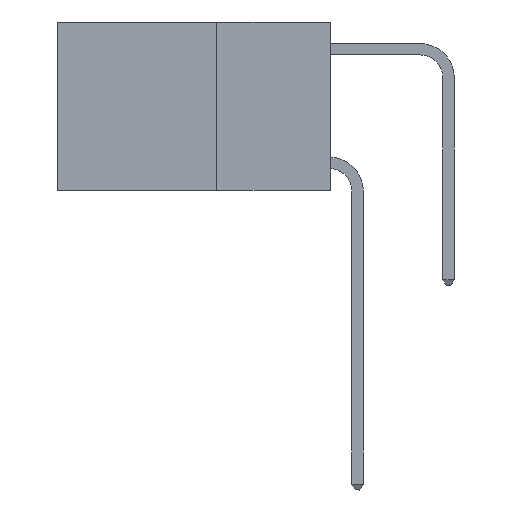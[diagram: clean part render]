
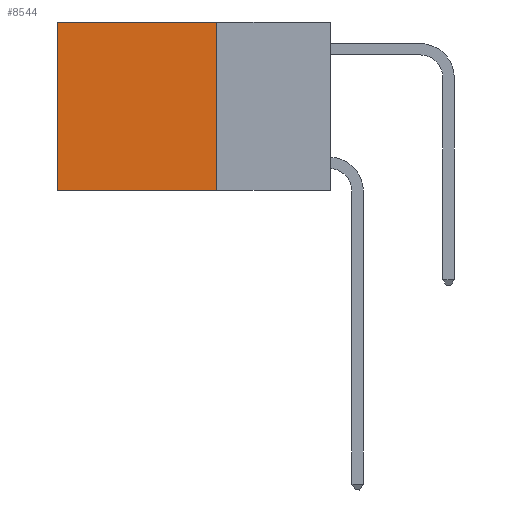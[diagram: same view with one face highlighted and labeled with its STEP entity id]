
A CAD part, left-side view. The second image highlights one B-rep face of the part: STEP entity #8544.
In plain terms, the highlighted planar face has unit normal (-1, 0, 0).
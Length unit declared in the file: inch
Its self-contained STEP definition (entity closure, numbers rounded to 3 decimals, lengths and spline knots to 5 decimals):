
#2169 = VECTOR ( 'NONE', #25110, 39.37008 ) ;
#2231 = ORIENTED_EDGE ( 'NONE', *, *, #23056, .T. ) ;
#2446 = CARTESIAN_POINT ( 'NONE',  ( 0.2625, 0.25, -0.37 ) ) ;
#4824 = LINE ( 'NONE', #13858, #25101 ) ;
#6864 = EDGE_LOOP ( 'NONE', ( #7836, #17168, #23738, #2231 ) ) ;
#6968 = CARTESIAN_POINT ( 'NONE',  ( 0.2625, 0.6, 0. ) ) ;
#7077 = LINE ( 'NONE', #13896, #2169 ) ;
#7836 = ORIENTED_EDGE ( 'NONE', *, *, #15672, .T. ) ;
#8544 = ADVANCED_FACE ( 'NONE', ( #14700 ), #27671, .F. ) ;
#9359 = CARTESIAN_POINT ( 'NONE',  ( 0.2625, 0.6, 0. ) ) ;
#9631 = LINE ( 'NONE', #6968, #21081 ) ;
#11119 = VECTOR ( 'NONE', #28921, 39.37008 ) ;
#11542 = VERTEX_POINT ( 'NONE', #9359 ) ;
#11868 = EDGE_CURVE ( 'NONE', #27145, #15104, #13313, .T. ) ;
#12349 = DIRECTION ( 'NONE',  ( 1., 0., 0. ) ) ;
#12414 = CARTESIAN_POINT ( 'NONE',  ( 0.2625, 0.6, -0.37 ) ) ;
#13313 = LINE ( 'NONE', #18003, #11119 ) ;
#13631 = DIRECTION ( 'NONE',  ( 0., 0., -1. ) ) ;
#13858 = CARTESIAN_POINT ( 'NONE',  ( 0.2625, 0.25, 0. ) ) ;
#13896 = CARTESIAN_POINT ( 'NONE',  ( 0.2625, 0.25, -0.37 ) ) ;
#14523 = VERTEX_POINT ( 'NONE', #12414 ) ;
#14700 = FACE_OUTER_BOUND ( 'NONE', #6864, .T. ) ;
#15104 = VERTEX_POINT ( 'NONE', #2446 ) ;
#15672 = EDGE_CURVE ( 'NONE', #11542, #14523, #9631, .T. ) ;
#16611 = CARTESIAN_POINT ( 'NONE',  ( 0.2625, 0.25, 0. ) ) ;
#17168 = ORIENTED_EDGE ( 'NONE', *, *, #25630, .F. ) ;
#18003 = CARTESIAN_POINT ( 'NONE',  ( 0.2625, 0.25, 0. ) ) ;
#19102 = DIRECTION ( 'NONE',  ( 0., 0., -1. ) ) ;
#20749 = DIRECTION ( 'NONE',  ( 0., 1., 0. ) ) ;
#21081 = VECTOR ( 'NONE', #13631, 39.37008 ) ;
#23056 = EDGE_CURVE ( 'NONE', #27145, #11542, #4824, .T. ) ;
#23738 = ORIENTED_EDGE ( 'NONE', *, *, #11868, .F. ) ;
#24439 = CARTESIAN_POINT ( 'NONE',  ( 0.2625, 0.25, 0. ) ) ;
#25101 = VECTOR ( 'NONE', #20749, 39.37008 ) ;
#25110 = DIRECTION ( 'NONE',  ( 0., 1., 0. ) ) ;
#25630 = EDGE_CURVE ( 'NONE', #15104, #14523, #7077, .T. ) ;
#26956 = AXIS2_PLACEMENT_3D ( 'NONE', #16611, #12349, #19102 ) ;
#27145 = VERTEX_POINT ( 'NONE', #24439 ) ;
#27671 = PLANE ( 'NONE',  #26956 ) ;
#28921 = DIRECTION ( 'NONE',  ( 0., 0., -1. ) ) ;
